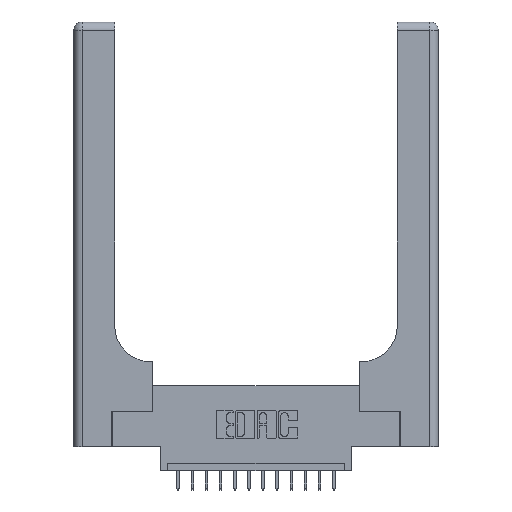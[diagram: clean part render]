
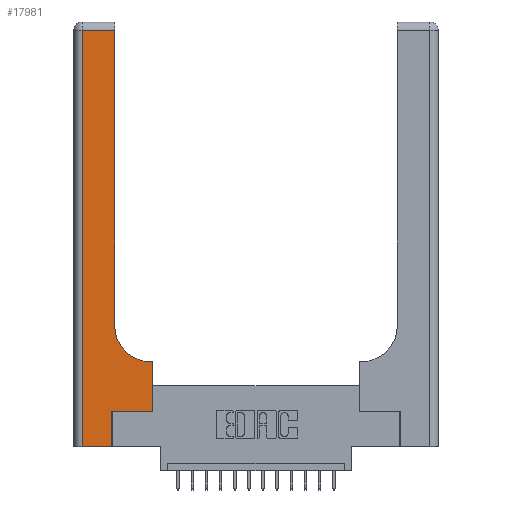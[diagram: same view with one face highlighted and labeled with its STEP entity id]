
A CAD part, top view. The second image highlights one B-rep face of the part: STEP entity #17981.
In plain terms, the highlighted planar face has unit normal (0, 0, 1).
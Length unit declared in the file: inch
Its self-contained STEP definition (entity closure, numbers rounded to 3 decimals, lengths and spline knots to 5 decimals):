
#69 = ORIENTED_EDGE ( 'NONE', *, *, #13359, .T. ) ;
#176 = VECTOR ( 'NONE', #12468, 39.37008 ) ;
#189 = ORIENTED_EDGE ( 'NONE', *, *, #5172, .T. ) ;
#416 = VERTEX_POINT ( 'NONE', #8663 ) ;
#558 = CARTESIAN_POINT ( 'NONE',  ( 0.06, 2.94, 0.37 ) ) ;
#742 = DIRECTION ( 'NONE',  ( 0., 0., -1. ) ) ;
#772 = AXIS2_PLACEMENT_3D ( 'NONE', #4030, #11227, #14125 ) ;
#1009 = CARTESIAN_POINT ( 'NONE',  ( 0.2915, 0.6, 0.37 ) ) ;
#1545 = LINE ( 'NONE', #4432, #7866 ) ;
#1648 = VERTEX_POINT ( 'NONE', #3330 ) ;
#1894 = ORIENTED_EDGE ( 'NONE', *, *, #6416, .T. ) ;
#2567 = VECTOR ( 'NONE', #16938, 39.37008 ) ;
#3056 = VERTEX_POINT ( 'NONE', #8123 ) ;
#3277 = EDGE_CURVE ( 'NONE', #3056, #10956, #10439, .T. ) ;
#3327 = ORIENTED_EDGE ( 'NONE', *, *, #5299, .T. ) ;
#3330 = CARTESIAN_POINT ( 'NONE',  ( 0.5585, 0.25, 0.37 ) ) ;
#3372 = DIRECTION ( 'NONE',  ( -1., 0., 0. ) ) ;
#3689 = CARTESIAN_POINT ( 'NONE',  ( 0.5415, 0.6, 0.37 ) ) ;
#3782 = VERTEX_POINT ( 'NONE', #16601 ) ;
#3802 = DIRECTION ( 'NONE',  ( 1., 0., 0. ) ) ;
#3897 = ORIENTED_EDGE ( 'NONE', *, *, #18154, .T. ) ;
#4027 = LINE ( 'NONE', #18226, #12699 ) ;
#4030 = CARTESIAN_POINT ( 'NONE',  ( 0.5415, 0.85, 0.37 ) ) ;
#4078 = CIRCLE ( 'NONE', #772, 0.25 ) ;
#4432 = CARTESIAN_POINT ( 'NONE',  ( 0., 2.94, 0.37 ) ) ;
#4484 = ORIENTED_EDGE ( 'NONE', *, *, #18174, .T. ) ;
#5172 = EDGE_CURVE ( 'NONE', #16873, #1648, #9583, .T. ) ;
#5299 = EDGE_CURVE ( 'NONE', #11960, #6350, #1545, .T. ) ;
#5365 = CARTESIAN_POINT ( 'NONE',  ( 0.269, 0., 0.37 ) ) ;
#5503 = CARTESIAN_POINT ( 'NONE',  ( 0.06, 3., 0.37 ) ) ;
#5968 = DIRECTION ( 'NONE',  ( 0., 1., 0. ) ) ;
#6161 = CARTESIAN_POINT ( 'NONE',  ( 0.269, 0., 0.37 ) ) ;
#6350 = VERTEX_POINT ( 'NONE', #558 ) ;
#6416 = EDGE_CURVE ( 'NONE', #1648, #3782, #4027, .T. ) ;
#6726 = VECTOR ( 'NONE', #12436, 39.37008 ) ;
#7866 = VECTOR ( 'NONE', #15658, 39.37008 ) ;
#8113 = LINE ( 'NONE', #1009, #6726 ) ;
#8123 = CARTESIAN_POINT ( 'NONE',  ( 0.06, 0., 0.37 ) ) ;
#8138 = CARTESIAN_POINT ( 'NONE',  ( 0.2915, 3., 0.37 ) ) ;
#8337 = DIRECTION ( 'NONE',  ( 0., 1., 0. ) ) ;
#8663 = CARTESIAN_POINT ( 'NONE',  ( 0.2915, 0.85, 0.37 ) ) ;
#8696 = CARTESIAN_POINT ( 'NONE',  ( 0.2915, 2.94, 0.37 ) ) ;
#8711 = VERTEX_POINT ( 'NONE', #3689 ) ;
#9498 = CARTESIAN_POINT ( 'NONE',  ( 0., 0., 0.37 ) ) ;
#9583 = LINE ( 'NONE', #10985, #15933 ) ;
#10439 = LINE ( 'NONE', #9498, #17081 ) ;
#10956 = VERTEX_POINT ( 'NONE', #5365 ) ;
#10985 = CARTESIAN_POINT ( 'NONE',  ( 0.269, 0.25, 0.37 ) ) ;
#11227 = DIRECTION ( 'NONE',  ( 0., 0., -1. ) ) ;
#11960 = VERTEX_POINT ( 'NONE', #8696 ) ;
#11986 = LINE ( 'NONE', #6161, #16833 ) ;
#12076 = PLANE ( 'NONE',  #17782 ) ;
#12408 = DIRECTION ( 'NONE',  ( 1., 0., 0. ) ) ;
#12436 = DIRECTION ( 'NONE',  ( -1., 0., 0. ) ) ;
#12468 = DIRECTION ( 'NONE',  ( 0., 1., 0. ) ) ;
#12699 = VECTOR ( 'NONE', #8337, 39.37008 ) ;
#12795 = ORIENTED_EDGE ( 'NONE', *, *, #15726, .T. ) ;
#12996 = LINE ( 'NONE', #5503, #2567 ) ;
#13359 = EDGE_CURVE ( 'NONE', #10956, #16873, #11986, .T. ) ;
#13950 = LINE ( 'NONE', #8138, #176 ) ;
#14125 = DIRECTION ( 'NONE',  ( 1., 0., 0. ) ) ;
#15506 = CARTESIAN_POINT ( 'NONE',  ( 0.269, 0.25, 0.37 ) ) ;
#15572 = ORIENTED_EDGE ( 'NONE', *, *, #3277, .T. ) ;
#15658 = DIRECTION ( 'NONE',  ( -1., 0., 0. ) ) ;
#15726 = EDGE_CURVE ( 'NONE', #6350, #3056, #12996, .T. ) ;
#15933 = VECTOR ( 'NONE', #12408, 39.37008 ) ;
#16283 = FACE_OUTER_BOUND ( 'NONE', #17806, .T. ) ;
#16454 = CARTESIAN_POINT ( 'NONE',  ( 0., 3., 0.37 ) ) ;
#16601 = CARTESIAN_POINT ( 'NONE',  ( 0.5585, 0.6, 0.37 ) ) ;
#16833 = VECTOR ( 'NONE', #5968, 39.37008 ) ;
#16873 = VERTEX_POINT ( 'NONE', #15506 ) ;
#16938 = DIRECTION ( 'NONE',  ( 0., -1., 0. ) ) ;
#17081 = VECTOR ( 'NONE', #3802, 39.37008 ) ;
#17394 = EDGE_CURVE ( 'NONE', #3782, #8711, #8113, .T. ) ;
#17782 = AXIS2_PLACEMENT_3D ( 'NONE', #16454, #742, #3372 ) ;
#17806 = EDGE_LOOP ( 'NONE', ( #4484, #3327, #12795, #15572, #69, #189, #1894, #18333, #3897 ) ) ;
#17981 = ADVANCED_FACE ( 'NONE', ( #16283 ), #12076, .F. ) ;
#18154 = EDGE_CURVE ( 'NONE', #8711, #416, #4078, .T. ) ;
#18174 = EDGE_CURVE ( 'NONE', #416, #11960, #13950, .T. ) ;
#18226 = CARTESIAN_POINT ( 'NONE',  ( 0.5585, 0.25, 0.37 ) ) ;
#18333 = ORIENTED_EDGE ( 'NONE', *, *, #17394, .T. ) ;
